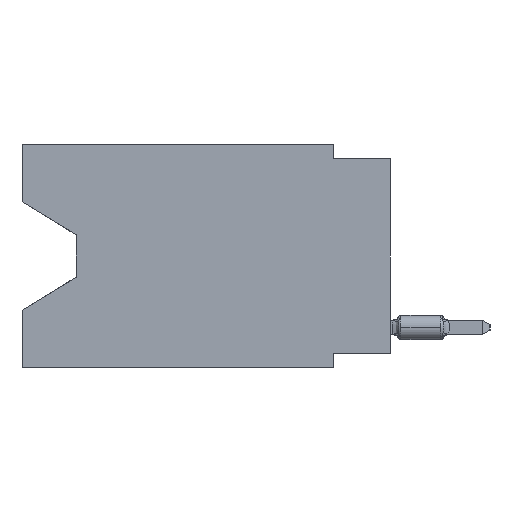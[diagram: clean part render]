
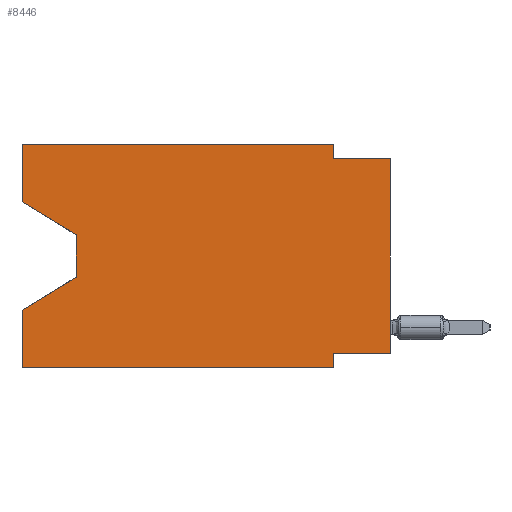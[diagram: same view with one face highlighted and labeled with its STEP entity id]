
A CAD part, left-side view. The second image highlights one B-rep face of the part: STEP entity #8446.
In plain terms, the highlighted planar face has unit normal (-1, 0, 0).
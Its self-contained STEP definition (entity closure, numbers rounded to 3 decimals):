
#282 = VERTEX_POINT ( 'NONE', #19284 ) ;
#366 = LINE ( 'NONE', #25186, #6907 ) ;
#452 = DIRECTION ( 'NONE',  ( 0., -1., 0. ) ) ;
#625 = DIRECTION ( 'NONE',  ( 0., -1., 0. ) ) ;
#1038 = VECTOR ( 'NONE', #20492, 1000. ) ;
#1039 = DIRECTION ( 'NONE',  ( 0., -0.855, -0.519 ) ) ;
#1422 = LINE ( 'NONE', #3867, #29761 ) ;
#1608 = ORIENTED_EDGE ( 'NONE', *, *, #10094, .F. ) ;
#1727 = EDGE_LOOP ( 'NONE', ( #13538, #2101, #31329, #15700, #6232, #1608, #11449, #1809, #6089, #39485, #32077, #32925 ) ) ;
#1809 = ORIENTED_EDGE ( 'NONE', *, *, #24175, .T. ) ;
#2101 = ORIENTED_EDGE ( 'NONE', *, *, #33899, .T. ) ;
#2663 = EDGE_CURVE ( 'NONE', #5323, #20265, #32453, .T. ) ;
#3715 = VERTEX_POINT ( 'NONE', #33012 ) ;
#3867 = CARTESIAN_POINT ( 'NONE',  ( 0., 0., -0.635 ) ) ;
#5122 = VERTEX_POINT ( 'NONE', #39730 ) ;
#5323 = VERTEX_POINT ( 'NONE', #20491 ) ;
#5669 = CARTESIAN_POINT ( 'NONE',  ( 0., 0., -0.635 ) ) ;
#6089 = ORIENTED_EDGE ( 'NONE', *, *, #17055, .F. ) ;
#6232 = ORIENTED_EDGE ( 'NONE', *, *, #35861, .T. ) ;
#6316 = EDGE_CURVE ( 'NONE', #14639, #27993, #25274, .T. ) ;
#6810 = VECTOR ( 'NONE', #452, 1000. ) ;
#6907 = VECTOR ( 'NONE', #34514, 1000. ) ;
#8446 = ADVANCED_FACE ( 'NONE', ( #35639 ), #20223, .F. ) ;
#9123 = DIRECTION ( 'NONE',  ( 0., 0., 1. ) ) ;
#9205 = CARTESIAN_POINT ( 'NONE',  ( 0., 16.383, 0. ) ) ;
#9258 = AXIS2_PLACEMENT_3D ( 'NONE', #11058, #26707, #17365 ) ;
#9358 = VECTOR ( 'NONE', #19880, 1000. ) ;
#9828 = CARTESIAN_POINT ( 'NONE',  ( 0., 16.383, -2.546 ) ) ;
#10094 = EDGE_CURVE ( 'NONE', #14789, #10874, #37711, .T. ) ;
#10874 = VERTEX_POINT ( 'NONE', #31068 ) ;
#10948 = VERTEX_POINT ( 'NONE', #16917 ) ;
#11058 = CARTESIAN_POINT ( 'NONE',  ( 0., 16.383, 0. ) ) ;
#11125 = CARTESIAN_POINT ( 'NONE',  ( 0., 13.97, -4.013 ) ) ;
#11141 = VERTEX_POINT ( 'NONE', #20547 ) ;
#11182 = VERTEX_POINT ( 'NONE', #5669 ) ;
#11339 = EDGE_CURVE ( 'NONE', #282, #20265, #366, .T. ) ;
#11449 = ORIENTED_EDGE ( 'NONE', *, *, #33719, .F. ) ;
#12050 = CARTESIAN_POINT ( 'NONE',  ( 0., 2.54, -9.271 ) ) ;
#12135 = CARTESIAN_POINT ( 'NONE',  ( 0., 2.54, -9.906 ) ) ;
#12772 = VECTOR ( 'NONE', #39898, 1000. ) ;
#12933 = DIRECTION ( 'NONE',  ( 0., 0., -1. ) ) ;
#13538 = ORIENTED_EDGE ( 'NONE', *, *, #6316, .T. ) ;
#14639 = VERTEX_POINT ( 'NONE', #22951 ) ;
#14789 = VERTEX_POINT ( 'NONE', #12050 ) ;
#15333 = VECTOR ( 'NONE', #37122, 1000. ) ;
#15700 = ORIENTED_EDGE ( 'NONE', *, *, #11339, .F. ) ;
#15904 = LINE ( 'NONE', #9205, #12772 ) ;
#16917 = CARTESIAN_POINT ( 'NONE',  ( 0., 16.383, 0. ) ) ;
#17055 = EDGE_CURVE ( 'NONE', #3715, #11182, #1422, .T. ) ;
#17365 = DIRECTION ( 'NONE',  ( 0., 0., -1. ) ) ;
#18342 = CARTESIAN_POINT ( 'NONE',  ( 0., 16.383, -7.36 ) ) ;
#19284 = CARTESIAN_POINT ( 'NONE',  ( 0., 16.383, -9.906 ) ) ;
#19880 = DIRECTION ( 'NONE',  ( 0., -1., 0. ) ) ;
#20080 = DIRECTION ( 'NONE',  ( 0., 0.855, -0.519 ) ) ;
#20223 = PLANE ( 'NONE',  #9258 ) ;
#20265 = VERTEX_POINT ( 'NONE', #18342 ) ;
#20491 = CARTESIAN_POINT ( 'NONE',  ( 0., 13.97, -5.893 ) ) ;
#20492 = DIRECTION ( 'NONE',  ( 0., 0., -1. ) ) ;
#20547 = CARTESIAN_POINT ( 'NONE',  ( 0., 0., -9.271 ) ) ;
#21550 = LINE ( 'NONE', #40019, #39113 ) ;
#21913 = CARTESIAN_POINT ( 'NONE',  ( 0., 2.54, 0. ) ) ;
#22294 = VECTOR ( 'NONE', #1039, 1000. ) ;
#22951 = CARTESIAN_POINT ( 'NONE',  ( 0., 16.383, -2.546 ) ) ;
#24175 = EDGE_CURVE ( 'NONE', #11141, #11182, #21550, .T. ) ;
#25186 = CARTESIAN_POINT ( 'NONE',  ( 0., 16.383, 0. ) ) ;
#25274 = LINE ( 'NONE', #9828, #22294 ) ;
#25541 = LINE ( 'NONE', #21913, #27126 ) ;
#25822 = CARTESIAN_POINT ( 'NONE',  ( 0., 13.97, -4.013 ) ) ;
#26363 = CARTESIAN_POINT ( 'NONE',  ( 0., 13.97, -5.893 ) ) ;
#26707 = DIRECTION ( 'NONE',  ( 1., 0., 0. ) ) ;
#26843 = LINE ( 'NONE', #29873, #36789 ) ;
#27126 = VECTOR ( 'NONE', #12933, 1000. ) ;
#27420 = VECTOR ( 'NONE', #20080, 1000. ) ;
#27993 = VERTEX_POINT ( 'NONE', #25822 ) ;
#28507 = LINE ( 'NONE', #34212, #6810 ) ;
#29003 = LINE ( 'NONE', #35297, #9358 ) ;
#29761 = VECTOR ( 'NONE', #625, 1000. ) ;
#29873 = CARTESIAN_POINT ( 'NONE',  ( 0., 0., -9.271 ) ) ;
#31068 = CARTESIAN_POINT ( 'NONE',  ( 0., 2.54, -9.906 ) ) ;
#31329 = ORIENTED_EDGE ( 'NONE', *, *, #2663, .T. ) ;
#32077 = ORIENTED_EDGE ( 'NONE', *, *, #36501, .F. ) ;
#32453 = LINE ( 'NONE', #26363, #27420 ) ;
#32925 = ORIENTED_EDGE ( 'NONE', *, *, #33506, .F. ) ;
#33012 = CARTESIAN_POINT ( 'NONE',  ( 0., 2.54, -0.635 ) ) ;
#33506 = EDGE_CURVE ( 'NONE', #14639, #10948, #15904, .T. ) ;
#33719 = EDGE_CURVE ( 'NONE', #11141, #14789, #26843, .T. ) ;
#33899 = EDGE_CURVE ( 'NONE', #27993, #5323, #38968, .T. ) ;
#34212 = CARTESIAN_POINT ( 'NONE',  ( 0., 16.383, 0. ) ) ;
#34514 = DIRECTION ( 'NONE',  ( 0., 0., 1. ) ) ;
#35293 = EDGE_CURVE ( 'NONE', #5122, #3715, #25541, .T. ) ;
#35297 = CARTESIAN_POINT ( 'NONE',  ( 0., 16.383, -9.906 ) ) ;
#35639 = FACE_OUTER_BOUND ( 'NONE', #1727, .T. ) ;
#35861 = EDGE_CURVE ( 'NONE', #282, #10874, #29003, .T. ) ;
#36501 = EDGE_CURVE ( 'NONE', #10948, #5122, #28507, .T. ) ;
#36789 = VECTOR ( 'NONE', #39042, 1000. ) ;
#37122 = DIRECTION ( 'NONE',  ( 0., 0., -1. ) ) ;
#37711 = LINE ( 'NONE', #12135, #15333 ) ;
#38968 = LINE ( 'NONE', #11125, #1038 ) ;
#39042 = DIRECTION ( 'NONE',  ( 0., 1., 0. ) ) ;
#39113 = VECTOR ( 'NONE', #9123, 1000. ) ;
#39485 = ORIENTED_EDGE ( 'NONE', *, *, #35293, .F. ) ;
#39730 = CARTESIAN_POINT ( 'NONE',  ( 0., 2.54, 0. ) ) ;
#39898 = DIRECTION ( 'NONE',  ( 0., 0., 1. ) ) ;
#40019 = CARTESIAN_POINT ( 'NONE',  ( 0., 0., 0. ) ) ;
